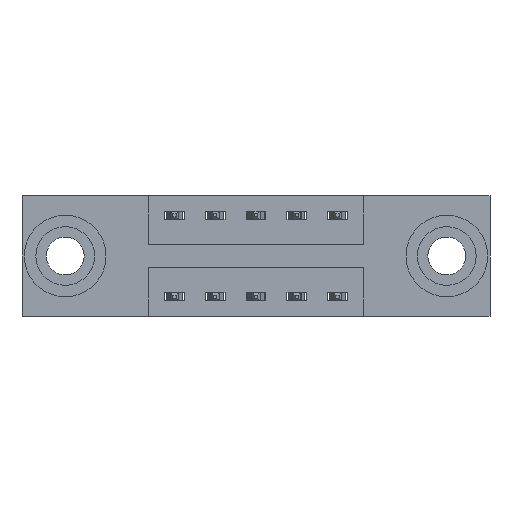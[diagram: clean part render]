
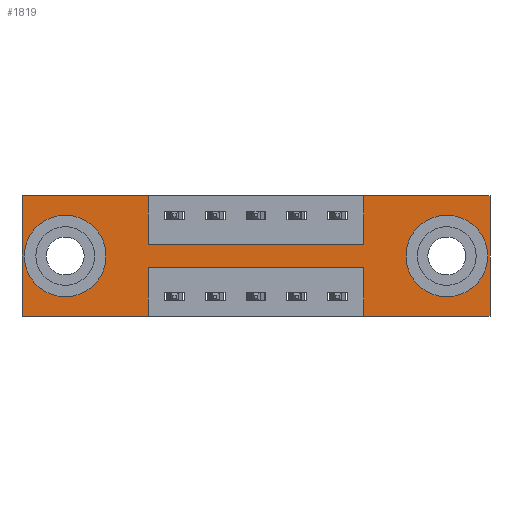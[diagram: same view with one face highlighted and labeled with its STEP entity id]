
A CAD part, front view. The second image highlights one B-rep face of the part: STEP entity #1819.
In plain terms, the highlighted planar face has unit normal (0, -1, 0).
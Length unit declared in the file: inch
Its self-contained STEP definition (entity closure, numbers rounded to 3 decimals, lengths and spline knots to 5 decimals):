
#201 = EDGE_CURVE ( 'NONE', #3635, #753, #4126, .T. ) ;
#225 = EDGE_CURVE ( 'NONE', #484, #6372, #5179, .T. ) ;
#425 = CARTESIAN_POINT ( 'NONE',  ( 0., 0., -0.37 ) ) ;
#429 = CIRCLE ( 'NONE', #3925, 0.078 ) ;
#447 = VECTOR ( 'NONE', #3428, 39.37008 ) ;
#450 = DIRECTION ( 'NONE',  ( 0., 0., 1. ) ) ;
#484 = VERTEX_POINT ( 'NONE', #3196 ) ;
#493 = CARTESIAN_POINT ( 'NONE',  ( 1.435, 0., 0. ) ) ;
#502 = ORIENTED_EDGE ( 'NONE', *, *, #2657, .F. ) ;
#538 = ORIENTED_EDGE ( 'NONE', *, *, #2885, .F. ) ;
#591 = DIRECTION ( 'NONE',  ( 0., 0., -1. ) ) ;
#601 = DIRECTION ( 'NONE',  ( 0., -1., 0. ) ) ;
#627 = CARTESIAN_POINT ( 'NONE',  ( 0.1325, 0., -0.107 ) ) ;
#670 = LINE ( 'NONE', #3561, #6853 ) ;
#703 = EDGE_CURVE ( 'NONE', #7355, #3635, #5605, .T. ) ;
#735 = VERTEX_POINT ( 'NONE', #3294 ) ;
#736 = CARTESIAN_POINT ( 'NONE',  ( 0.3875, 0., -0.22 ) ) ;
#753 = VERTEX_POINT ( 'NONE', #6445 ) ;
#799 = CARTESIAN_POINT ( 'NONE',  ( 1.3025, 0., -0.263 ) ) ;
#933 = EDGE_CURVE ( 'NONE', #9206, #4432, #7129, .T. ) ;
#982 = EDGE_CURVE ( 'NONE', #6372, #9206, #6837, .T. ) ;
#997 = VECTOR ( 'NONE', #2761, 39.37008 ) ;
#1003 = CIRCLE ( 'NONE', #2241, 0.078 ) ;
#1022 = DIRECTION ( 'NONE',  ( 0., 1., 0. ) ) ;
#1106 = VERTEX_POINT ( 'NONE', #6318 ) ;
#1301 = CARTESIAN_POINT ( 'NONE',  ( 0., 0., 0. ) ) ;
#1316 = LINE ( 'NONE', #493, #1769 ) ;
#1425 = CARTESIAN_POINT ( 'NONE',  ( 0., 0., -0.37 ) ) ;
#1639 = AXIS2_PLACEMENT_3D ( 'NONE', #5988, #5070, #8648 ) ;
#1769 = VECTOR ( 'NONE', #8412, 39.37008 ) ;
#1809 = CARTESIAN_POINT ( 'NONE',  ( 1.3025, 0., -0.185 ) ) ;
#1819 = ADVANCED_FACE ( 'NONE', ( #8620, #2883, #4225 ), #7897, .T. ) ;
#1847 = DIRECTION ( 'NONE',  ( 0., 0., 1. ) ) ;
#1870 = ORIENTED_EDGE ( 'NONE', *, *, #6109, .F. ) ;
#2035 = VERTEX_POINT ( 'NONE', #3406 ) ;
#2241 = AXIS2_PLACEMENT_3D ( 'NONE', #1809, #1022, #6108 ) ;
#2303 = ORIENTED_EDGE ( 'NONE', *, *, #4524, .F. ) ;
#2622 = VERTEX_POINT ( 'NONE', #1301 ) ;
#2657 = EDGE_CURVE ( 'NONE', #3705, #2622, #670, .T. ) ;
#2761 = DIRECTION ( 'NONE',  ( 1., 0., 0. ) ) ;
#2778 = CARTESIAN_POINT ( 'NONE',  ( 0.3875, 0., -0.15 ) ) ;
#2799 = DIRECTION ( 'NONE',  ( 0., 0., 1. ) ) ;
#2883 = FACE_BOUND ( 'NONE', #8587, .T. ) ;
#2885 = EDGE_CURVE ( 'NONE', #4432, #3705, #5522, .T. ) ;
#3131 = CARTESIAN_POINT ( 'NONE',  ( 0.1325, 0., -0.263 ) ) ;
#3196 = CARTESIAN_POINT ( 'NONE',  ( 1.0475, 0., -0.37 ) ) ;
#3231 = ORIENTED_EDGE ( 'NONE', *, *, #6603, .T. ) ;
#3238 = VECTOR ( 'NONE', #3394, 39.37008 ) ;
#3239 = VERTEX_POINT ( 'NONE', #799 ) ;
#3263 = ORIENTED_EDGE ( 'NONE', *, *, #4565, .T. ) ;
#3294 = CARTESIAN_POINT ( 'NONE',  ( 1.435, 0., -0.37 ) ) ;
#3383 = CARTESIAN_POINT ( 'NONE',  ( 1.0475, 0., 0. ) ) ;
#3394 = DIRECTION ( 'NONE',  ( 1., 0., 0. ) ) ;
#3406 = CARTESIAN_POINT ( 'NONE',  ( 1.435, 0., 0. ) ) ;
#3428 = DIRECTION ( 'NONE',  ( -1., 0., 0. ) ) ;
#3461 = DIRECTION ( 'NONE',  ( 0., 0., -1. ) ) ;
#3477 = CARTESIAN_POINT ( 'NONE',  ( 0., 0., -0.37 ) ) ;
#3555 = CARTESIAN_POINT ( 'NONE',  ( 1.3025, 0., -0.185 ) ) ;
#3561 = CARTESIAN_POINT ( 'NONE',  ( 0., 0., 0. ) ) ;
#3635 = VERTEX_POINT ( 'NONE', #5196 ) ;
#3641 = DIRECTION ( 'NONE',  ( 0., 0., 1. ) ) ;
#3705 = VERTEX_POINT ( 'NONE', #3477 ) ;
#3872 = VECTOR ( 'NONE', #591, 39.37008 ) ;
#3925 = AXIS2_PLACEMENT_3D ( 'NONE', #3555, #5002, #3461 ) ;
#4021 = CARTESIAN_POINT ( 'NONE',  ( 0., 0., -0.37 ) ) ;
#4126 = LINE ( 'NONE', #2778, #3238 ) ;
#4155 = DIRECTION ( 'NONE',  ( 0., 1., 0. ) ) ;
#4156 = EDGE_CURVE ( 'NONE', #735, #484, #5503, .T. ) ;
#4162 = EDGE_CURVE ( 'NONE', #753, #1106, #8319, .T. ) ;
#4175 = ORIENTED_EDGE ( 'NONE', *, *, #933, .F. ) ;
#4193 = VECTOR ( 'NONE', #7837, 39.37008 ) ;
#4225 = FACE_OUTER_BOUND ( 'NONE', #4458, .T. ) ;
#4281 = EDGE_CURVE ( 'NONE', #7328, #4415, #7238, .T. ) ;
#4415 = VERTEX_POINT ( 'NONE', #3131 ) ;
#4432 = VERTEX_POINT ( 'NONE', #4724 ) ;
#4458 = EDGE_LOOP ( 'NONE', ( #4175, #7564, #8486, #8097, #7849, #1870, #4513, #9103, #7057, #2303, #502, #538 ) ) ;
#4513 = ORIENTED_EDGE ( 'NONE', *, *, #4162, .F. ) ;
#4524 = EDGE_CURVE ( 'NONE', #2622, #7355, #8962, .T. ) ;
#4565 = EDGE_CURVE ( 'NONE', #3239, #6385, #429, .T. ) ;
#4724 = CARTESIAN_POINT ( 'NONE',  ( 0.3875, 0., -0.37 ) ) ;
#4965 = CARTESIAN_POINT ( 'NONE',  ( 0.3875, 0., 0. ) ) ;
#5002 = DIRECTION ( 'NONE',  ( 0., 1., 0. ) ) ;
#5070 = DIRECTION ( 'NONE',  ( 0., 1., 0. ) ) ;
#5179 = LINE ( 'NONE', #8032, #8084 ) ;
#5196 = CARTESIAN_POINT ( 'NONE',  ( 0.3875, 0., -0.15 ) ) ;
#5387 = CARTESIAN_POINT ( 'NONE',  ( 0., 0., 0. ) ) ;
#5503 = LINE ( 'NONE', #4021, #447 ) ;
#5522 = LINE ( 'NONE', #425, #7157 ) ;
#5595 = CARTESIAN_POINT ( 'NONE',  ( 0.3875, 0., -0.37 ) ) ;
#5605 = LINE ( 'NONE', #9139, #3872 ) ;
#5793 = DIRECTION ( 'NONE',  ( 0., 0., -1. ) ) ;
#5879 = CARTESIAN_POINT ( 'NONE',  ( 1.0475, 0., -0.22 ) ) ;
#5988 = CARTESIAN_POINT ( 'NONE',  ( 0.1325, 0., -0.185 ) ) ;
#6108 = DIRECTION ( 'NONE',  ( 0., 0., -1. ) ) ;
#6109 = EDGE_CURVE ( 'NONE', #1106, #2035, #8016, .T. ) ;
#6318 = CARTESIAN_POINT ( 'NONE',  ( 1.0475, 0., 0. ) ) ;
#6372 = VERTEX_POINT ( 'NONE', #5879 ) ;
#6378 = VECTOR ( 'NONE', #450, 39.37008 ) ;
#6385 = VERTEX_POINT ( 'NONE', #6509 ) ;
#6445 = CARTESIAN_POINT ( 'NONE',  ( 1.0475, 0., -0.15 ) ) ;
#6469 = CIRCLE ( 'NONE', #7359, 0.078 ) ;
#6509 = CARTESIAN_POINT ( 'NONE',  ( 1.3025, 0., -0.107 ) ) ;
#6603 = EDGE_CURVE ( 'NONE', #6385, #3239, #1003, .T. ) ;
#6767 = EDGE_CURVE ( 'NONE', #2035, #735, #1316, .T. ) ;
#6837 = LINE ( 'NONE', #736, #7806 ) ;
#6853 = VECTOR ( 'NONE', #2799, 39.37008 ) ;
#7057 = ORIENTED_EDGE ( 'NONE', *, *, #703, .F. ) ;
#7078 = CARTESIAN_POINT ( 'NONE',  ( 0., 0., 0. ) ) ;
#7129 = LINE ( 'NONE', #5595, #4193 ) ;
#7157 = VECTOR ( 'NONE', #8425, 39.37008 ) ;
#7189 = EDGE_CURVE ( 'NONE', #4415, #7328, #6469, .T. ) ;
#7238 = CIRCLE ( 'NONE', #1639, 0.078 ) ;
#7328 = VERTEX_POINT ( 'NONE', #627 ) ;
#7355 = VERTEX_POINT ( 'NONE', #4965 ) ;
#7359 = AXIS2_PLACEMENT_3D ( 'NONE', #8449, #4155, #1847 ) ;
#7564 = ORIENTED_EDGE ( 'NONE', *, *, #982, .F. ) ;
#7697 = EDGE_LOOP ( 'NONE', ( #3231, #3263 ) ) ;
#7806 = VECTOR ( 'NONE', #8159, 39.37008 ) ;
#7837 = DIRECTION ( 'NONE',  ( 0., 0., -1. ) ) ;
#7849 = ORIENTED_EDGE ( 'NONE', *, *, #6767, .F. ) ;
#7897 = PLANE ( 'NONE',  #9149 ) ;
#8016 = LINE ( 'NONE', #7078, #997 ) ;
#8032 = CARTESIAN_POINT ( 'NONE',  ( 1.0475, 0., -0.37 ) ) ;
#8084 = VECTOR ( 'NONE', #3641, 39.37008 ) ;
#8097 = ORIENTED_EDGE ( 'NONE', *, *, #4156, .F. ) ;
#8110 = ORIENTED_EDGE ( 'NONE', *, *, #7189, .T. ) ;
#8159 = DIRECTION ( 'NONE',  ( -1., 0., 0. ) ) ;
#8243 = DIRECTION ( 'NONE',  ( 1., 0., 0. ) ) ;
#8319 = LINE ( 'NONE', #3383, #6378 ) ;
#8412 = DIRECTION ( 'NONE',  ( 0., 0., -1. ) ) ;
#8425 = DIRECTION ( 'NONE',  ( -1., 0., 0. ) ) ;
#8449 = CARTESIAN_POINT ( 'NONE',  ( 0.1325, 0., -0.185 ) ) ;
#8486 = ORIENTED_EDGE ( 'NONE', *, *, #225, .F. ) ;
#8587 = EDGE_LOOP ( 'NONE', ( #8955, #8110 ) ) ;
#8620 = FACE_BOUND ( 'NONE', #7697, .T. ) ;
#8648 = DIRECTION ( 'NONE',  ( 0., 0., 1. ) ) ;
#8955 = ORIENTED_EDGE ( 'NONE', *, *, #4281, .T. ) ;
#8962 = LINE ( 'NONE', #5387, #9070 ) ;
#9070 = VECTOR ( 'NONE', #8243, 39.37008 ) ;
#9075 = CARTESIAN_POINT ( 'NONE',  ( 0.3875, 0., -0.22 ) ) ;
#9103 = ORIENTED_EDGE ( 'NONE', *, *, #201, .F. ) ;
#9139 = CARTESIAN_POINT ( 'NONE',  ( 0.3875, 0., 0. ) ) ;
#9149 = AXIS2_PLACEMENT_3D ( 'NONE', #1425, #601, #5793 ) ;
#9206 = VERTEX_POINT ( 'NONE', #9075 ) ;
